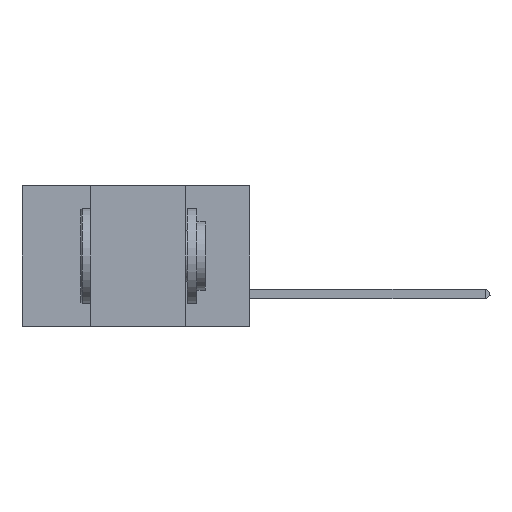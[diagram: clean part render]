
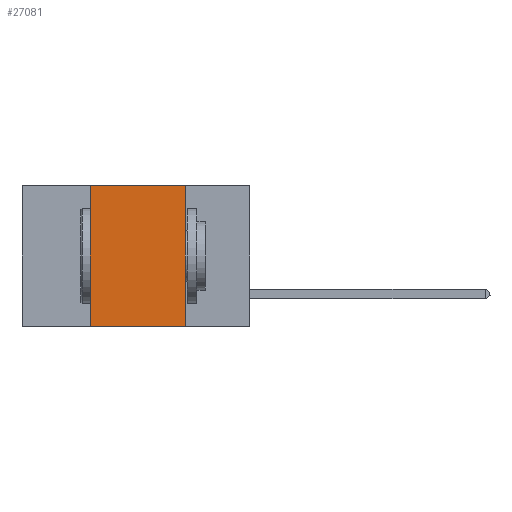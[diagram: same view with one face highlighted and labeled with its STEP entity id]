
A CAD part, left-side view. The second image highlights one B-rep face of the part: STEP entity #27081.
In plain terms, the highlighted planar face has unit normal (-1, 0, 0).
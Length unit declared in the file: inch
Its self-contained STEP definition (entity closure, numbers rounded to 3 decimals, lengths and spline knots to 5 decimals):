
#1053 = VERTEX_POINT ( 'NONE', #14927 ) ;
#1941 = VECTOR ( 'NONE', #35067, 39.37008 ) ;
#3025 = ORIENTED_EDGE ( 'NONE', *, *, #15158, .F. ) ;
#4086 = LINE ( 'NONE', #27761, #30094 ) ;
#4205 = CARTESIAN_POINT ( 'NONE',  ( 0., 0.6, 0. ) ) ;
#5024 = CARTESIAN_POINT ( 'NONE',  ( 0., 0.42, -0.37 ) ) ;
#6026 = EDGE_CURVE ( 'NONE', #20076, #1053, #10635, .T. ) ;
#6089 = DIRECTION ( 'NONE',  ( 0., -1., 0. ) ) ;
#8349 = CARTESIAN_POINT ( 'NONE',  ( 0., 0.42, 0. ) ) ;
#9724 = EDGE_LOOP ( 'NONE', ( #17667, #3025, #38031, #17452 ) ) ;
#10488 = CARTESIAN_POINT ( 'NONE',  ( 0., 0.17, 0. ) ) ;
#10635 = LINE ( 'NONE', #10488, #1941 ) ;
#11758 = DIRECTION ( 'NONE',  ( 0., 0., -1. ) ) ;
#12655 = VERTEX_POINT ( 'NONE', #20373 ) ;
#14059 = LINE ( 'NONE', #4205, #34259 ) ;
#14862 = CARTESIAN_POINT ( 'NONE',  ( 0., 0.6, 0. ) ) ;
#14927 = CARTESIAN_POINT ( 'NONE',  ( 0., 0.17, -0.37 ) ) ;
#15158 = EDGE_CURVE ( 'NONE', #12655, #20076, #14059, .T. ) ;
#16088 = FACE_OUTER_BOUND ( 'NONE', #9724, .T. ) ;
#17452 = ORIENTED_EDGE ( 'NONE', *, *, #32178, .T. ) ;
#17667 = ORIENTED_EDGE ( 'NONE', *, *, #6026, .F. ) ;
#20076 = VERTEX_POINT ( 'NONE', #25555 ) ;
#20091 = AXIS2_PLACEMENT_3D ( 'NONE', #14862, #36053, #11758 ) ;
#20373 = CARTESIAN_POINT ( 'NONE',  ( 0., 0.42, 0. ) ) ;
#23953 = DIRECTION ( 'NONE',  ( 0., 0., 1. ) ) ;
#24455 = LINE ( 'NONE', #8349, #35531 ) ;
#25555 = CARTESIAN_POINT ( 'NONE',  ( 0., 0.17, 0. ) ) ;
#27081 = ADVANCED_FACE ( 'NONE', ( #16088 ), #29798, .F. ) ;
#27761 = CARTESIAN_POINT ( 'NONE',  ( 0., 0.6, -0.37 ) ) ;
#29798 = PLANE ( 'NONE',  #20091 ) ;
#30094 = VECTOR ( 'NONE', #6089, 39.37008 ) ;
#31660 = DIRECTION ( 'NONE',  ( 0., -1., 0. ) ) ;
#32178 = EDGE_CURVE ( 'NONE', #36927, #1053, #4086, .T. ) ;
#34259 = VECTOR ( 'NONE', #31660, 39.37008 ) ;
#35067 = DIRECTION ( 'NONE',  ( 0., 0., -1. ) ) ;
#35531 = VECTOR ( 'NONE', #23953, 39.37008 ) ;
#36053 = DIRECTION ( 'NONE',  ( 1., 0., 0. ) ) ;
#36137 = EDGE_CURVE ( 'NONE', #36927, #12655, #24455, .T. ) ;
#36927 = VERTEX_POINT ( 'NONE', #5024 ) ;
#38031 = ORIENTED_EDGE ( 'NONE', *, *, #36137, .F. ) ;
